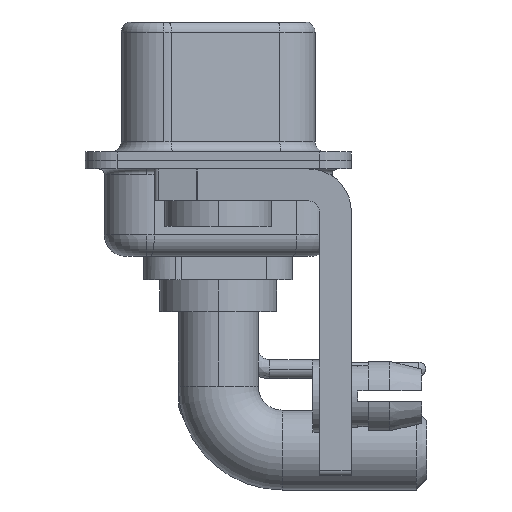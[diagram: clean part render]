
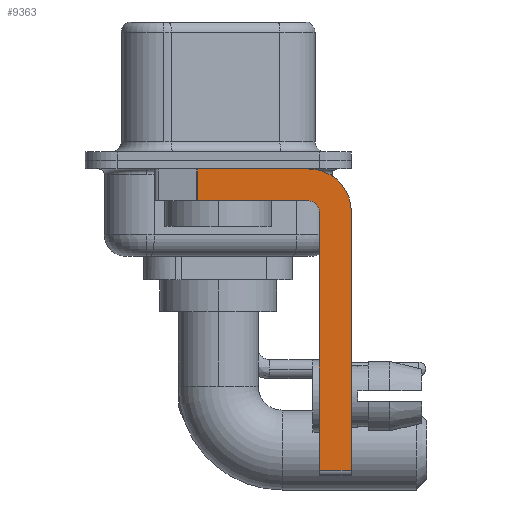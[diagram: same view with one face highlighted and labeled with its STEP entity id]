
A CAD part, left-side view. The second image highlights one B-rep face of the part: STEP entity #9363.
In plain terms, the highlighted planar face has unit normal (-1, 0, 0).
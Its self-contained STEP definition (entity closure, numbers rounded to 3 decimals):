
#90 = DIRECTION ( 'NONE',  ( -1., 0., 0. ) ) ;
#454 = DIRECTION ( 'NONE',  ( 0., 0., -1. ) ) ;
#1133 = CARTESIAN_POINT ( 'NONE',  ( -2.9, -4.25, -1.9 ) ) ;
#1257 = DIRECTION ( 'NONE',  ( 0., 1., 0. ) ) ;
#2230 = CARTESIAN_POINT ( 'NONE',  ( -2.9, -4.75, -2.4 ) ) ;
#2349 = VERTEX_POINT ( 'NONE', #4382 ) ;
#2618 = EDGE_CURVE ( 'NONE', #20159, #14911, #15499, .T. ) ;
#3214 = ORIENTED_EDGE ( 'NONE', *, *, #7215, .T. ) ;
#3342 = CARTESIAN_POINT ( 'NONE',  ( -2.9, -4.25, -14.55 ) ) ;
#4170 = VECTOR ( 'NONE', #1257, 1000. ) ;
#4252 = CARTESIAN_POINT ( 'NONE',  ( -2.9, -4.75, -14.8 ) ) ;
#4376 = CARTESIAN_POINT ( 'NONE',  ( -2.9, -4.25, -0.4 ) ) ;
#4382 = CARTESIAN_POINT ( 'NONE',  ( -2.9, 0.978, -1.9 ) ) ;
#4474 = CARTESIAN_POINT ( 'NONE',  ( -2.9, -4.25, -1.9 ) ) ;
#4643 = VERTEX_POINT ( 'NONE', #13791 ) ;
#4990 = DIRECTION ( 'NONE',  ( 0., -1., 0. ) ) ;
#5587 = DIRECTION ( 'NONE',  ( 0., 0., -1. ) ) ;
#5842 = PLANE ( 'NONE',  #9743 ) ;
#6919 = LINE ( 'NONE', #22251, #13029 ) ;
#7215 = EDGE_CURVE ( 'NONE', #12785, #2349, #21218, .T. ) ;
#7370 = EDGE_CURVE ( 'NONE', #15039, #4643, #8784, .T. ) ;
#7473 = CARTESIAN_POINT ( 'NONE',  ( -2.9, -6.25, -2.4 ) ) ;
#7493 = FACE_OUTER_BOUND ( 'NONE', #20312, .T. ) ;
#7729 = EDGE_CURVE ( 'NONE', #11906, #2349, #20119, .T. ) ;
#8053 = LINE ( 'NONE', #7473, #10912 ) ;
#8084 = ORIENTED_EDGE ( 'NONE', *, *, #22397, .F. ) ;
#8784 = LINE ( 'NONE', #3342, #17468 ) ;
#9166 = DIRECTION ( 'NONE',  ( 1., 0., 0. ) ) ;
#9363 = ADVANCED_FACE ( 'NONE', ( #7493 ), #5842, .F. ) ;
#9670 = CARTESIAN_POINT ( 'NONE',  ( -2.9, -4.25, -2.4 ) ) ;
#9743 = AXIS2_PLACEMENT_3D ( 'NONE', #17111, #24839, #5587 ) ;
#9749 = VERTEX_POINT ( 'NONE', #2230 ) ;
#10912 = VECTOR ( 'NONE', #24818, 1000. ) ;
#11365 = ORIENTED_EDGE ( 'NONE', *, *, #7370, .T. ) ;
#11833 = LINE ( 'NONE', #4252, #13350 ) ;
#11906 = VERTEX_POINT ( 'NONE', #4474 ) ;
#11955 = DIRECTION ( 'NONE',  ( 0., 0., 1. ) ) ;
#12785 = VERTEX_POINT ( 'NONE', #23701 ) ;
#12954 = CARTESIAN_POINT ( 'NONE',  ( -2.9, -4.25, -2.4 ) ) ;
#13029 = VECTOR ( 'NONE', #14767, 1000. ) ;
#13058 = ORIENTED_EDGE ( 'NONE', *, *, #22082, .F. ) ;
#13270 = VECTOR ( 'NONE', #454, 1000. ) ;
#13350 = VECTOR ( 'NONE', #11955, 1000. ) ;
#13791 = CARTESIAN_POINT ( 'NONE',  ( -2.9, -6.25, -14.55 ) ) ;
#14126 = CARTESIAN_POINT ( 'NONE',  ( -2.9, -4.75, -14.55 ) ) ;
#14272 = AXIS2_PLACEMENT_3D ( 'NONE', #12954, #9166, #24619 ) ;
#14767 = DIRECTION ( 'NONE',  ( 0., -1., 0. ) ) ;
#14911 = VERTEX_POINT ( 'NONE', #23162 ) ;
#15014 = DIRECTION ( 'NONE',  ( 0., 0., 1. ) ) ;
#15039 = VERTEX_POINT ( 'NONE', #14126 ) ;
#15499 = CIRCLE ( 'NONE', #14272, 2. ) ;
#15553 = ORIENTED_EDGE ( 'NONE', *, *, #21636, .F. ) ;
#15746 = CARTESIAN_POINT ( 'NONE',  ( -2.9, 0.978, -1.9 ) ) ;
#17111 = CARTESIAN_POINT ( 'NONE',  ( -2.9, -4.25, -2.4 ) ) ;
#17468 = VECTOR ( 'NONE', #4990, 1000. ) ;
#17720 = EDGE_CURVE ( 'NONE', #14911, #4643, #8053, .T. ) ;
#18706 = ORIENTED_EDGE ( 'NONE', *, *, #7729, .F. ) ;
#19019 = CIRCLE ( 'NONE', #19410, 0.5 ) ;
#19410 = AXIS2_PLACEMENT_3D ( 'NONE', #9670, #90, #15014 ) ;
#20119 = LINE ( 'NONE', #1133, #4170 ) ;
#20159 = VERTEX_POINT ( 'NONE', #4376 ) ;
#20312 = EDGE_LOOP ( 'NONE', ( #15553, #3214, #18706, #8084, #13058, #11365, #23849, #23182 ) ) ;
#21218 = LINE ( 'NONE', #15746, #13270 ) ;
#21636 = EDGE_CURVE ( 'NONE', #12785, #20159, #6919, .T. ) ;
#22082 = EDGE_CURVE ( 'NONE', #15039, #9749, #11833, .T. ) ;
#22251 = CARTESIAN_POINT ( 'NONE',  ( -2.9, 3., -0.4 ) ) ;
#22397 = EDGE_CURVE ( 'NONE', #9749, #11906, #19019, .T. ) ;
#23162 = CARTESIAN_POINT ( 'NONE',  ( -2.9, -6.25, -2.4 ) ) ;
#23182 = ORIENTED_EDGE ( 'NONE', *, *, #2618, .F. ) ;
#23701 = CARTESIAN_POINT ( 'NONE',  ( -2.9, 0.978, -0.4 ) ) ;
#23849 = ORIENTED_EDGE ( 'NONE', *, *, #17720, .F. ) ;
#24619 = DIRECTION ( 'NONE',  ( 0., 0., -1. ) ) ;
#24818 = DIRECTION ( 'NONE',  ( 0., 0., -1. ) ) ;
#24839 = DIRECTION ( 'NONE',  ( 1., 0., 0. ) ) ;
